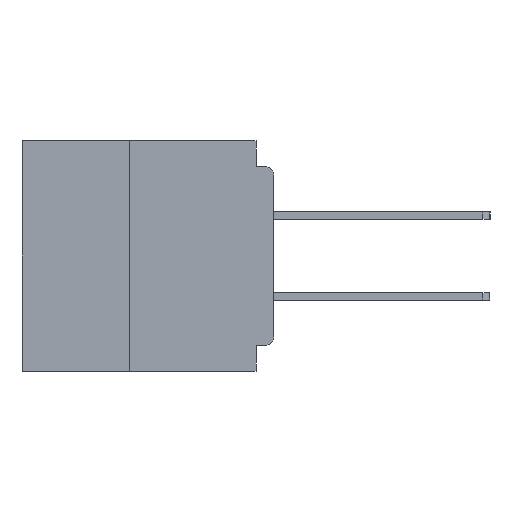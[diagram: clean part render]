
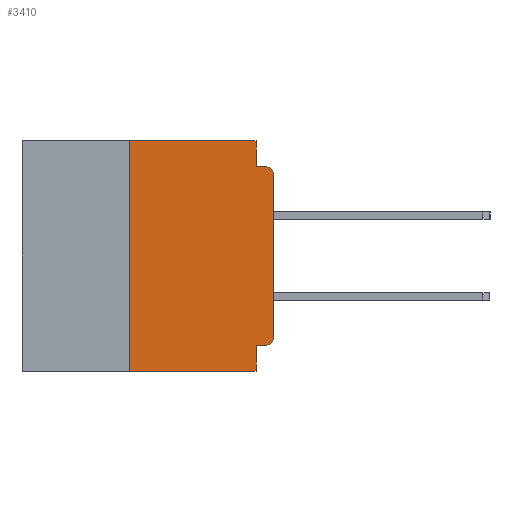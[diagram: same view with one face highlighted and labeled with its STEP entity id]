
A CAD part, left-side view. The second image highlights one B-rep face of the part: STEP entity #3410.
In plain terms, the highlighted planar face has unit normal (-1, 0, 0).
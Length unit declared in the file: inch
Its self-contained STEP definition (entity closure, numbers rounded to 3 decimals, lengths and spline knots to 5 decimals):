
#712 = EDGE_CURVE ( 'NONE', #41883, #41600, #4166, .T. ) ;
#961 = VERTEX_POINT ( 'NONE', #9339 ) ;
#2722 = VECTOR ( 'NONE', #60346, 39.37008 ) ;
#3410 = ADVANCED_FACE ( 'NONE', ( #14158 ), #40095, .F. ) ;
#4166 = CIRCLE ( 'NONE', #54427, 0.015 ) ;
#4264 = LINE ( 'NONE', #10552, #2722 ) ;
#5051 = CARTESIAN_POINT ( 'NONE',  ( 0., 0., -0.34 ) ) ;
#5794 = EDGE_CURVE ( 'NONE', #13918, #59047, #13014, .T. ) ;
#7141 = EDGE_LOOP ( 'NONE', ( #13657, #13725, #13972, #15127, #15291, #16642, #16858, #16979, #18380, #18443 ) ) ;
#9001 = VECTOR ( 'NONE', #41892, 39.37008 ) ;
#9339 = CARTESIAN_POINT ( 'NONE',  ( 0., 0.031, -0.045 ) ) ;
#10482 = VECTOR ( 'NONE', #23053, 39.37008 ) ;
#10552 = CARTESIAN_POINT ( 'NONE',  ( 0., 0., -0.045 ) ) ;
#12999 = CARTESIAN_POINT ( 'NONE',  ( 0., 0., 0. ) ) ;
#13014 = LINE ( 'NONE', #35669, #51040 ) ;
#13310 = CARTESIAN_POINT ( 'NONE',  ( 0., 0.437, 0. ) ) ;
#13657 = ORIENTED_EDGE ( 'NONE', *, *, #55321, .T. ) ;
#13725 = ORIENTED_EDGE ( 'NONE', *, *, #25751, .T. ) ;
#13918 = VERTEX_POINT ( 'NONE', #22809 ) ;
#13972 = ORIENTED_EDGE ( 'NONE', *, *, #45999, .F. ) ;
#14158 = FACE_OUTER_BOUND ( 'NONE', #7141, .T. ) ;
#14309 = CARTESIAN_POINT ( 'NONE',  ( 0., 0.25, -0.4 ) ) ;
#15127 = ORIENTED_EDGE ( 'NONE', *, *, #40998, .F. ) ;
#15291 = ORIENTED_EDGE ( 'NONE', *, *, #24713, .F. ) ;
#16642 = ORIENTED_EDGE ( 'NONE', *, *, #40316, .F. ) ;
#16858 = ORIENTED_EDGE ( 'NONE', *, *, #39664, .T. ) ;
#16963 = CARTESIAN_POINT ( 'NONE',  ( 0., 0.015, -0.355 ) ) ;
#16979 = ORIENTED_EDGE ( 'NONE', *, *, #5794, .F. ) ;
#17107 = CARTESIAN_POINT ( 'NONE',  ( 0., 0., -0.355 ) ) ;
#18256 = AXIS2_PLACEMENT_3D ( 'NONE', #50544, #20895, #55479 ) ;
#18380 = ORIENTED_EDGE ( 'NONE', *, *, #43912, .F. ) ;
#18443 = ORIENTED_EDGE ( 'NONE', *, *, #712, .T. ) ;
#19153 = VERTEX_POINT ( 'NONE', #29732 ) ;
#20151 = CARTESIAN_POINT ( 'NONE',  ( 0., 0.031, 0. ) ) ;
#20895 = DIRECTION ( 'NONE',  ( -1., 0., 0. ) ) ;
#21794 = VERTEX_POINT ( 'NONE', #53941 ) ;
#21853 = VECTOR ( 'NONE', #34099, 39.37008 ) ;
#22424 = VECTOR ( 'NONE', #33102, 39.37008 ) ;
#22809 = CARTESIAN_POINT ( 'NONE',  ( 0., 0.031, -0.355 ) ) ;
#23053 = DIRECTION ( 'NONE',  ( 0., 0., 1. ) ) ;
#23992 = LINE ( 'NONE', #13310, #22424 ) ;
#24713 = EDGE_CURVE ( 'NONE', #21794, #55453, #23992, .T. ) ;
#25751 = EDGE_CURVE ( 'NONE', #19153, #29662, #40828, .T. ) ;
#25863 = LINE ( 'NONE', #28375, #49073 ) ;
#28375 = CARTESIAN_POINT ( 'NONE',  ( 0., 0.437, -0.4 ) ) ;
#28702 = CARTESIAN_POINT ( 'NONE',  ( 0., 0.031, -0.4 ) ) ;
#29662 = VERTEX_POINT ( 'NONE', #58055 ) ;
#29732 = CARTESIAN_POINT ( 'NONE',  ( 0., 0., -0.06 ) ) ;
#33102 = DIRECTION ( 'NONE',  ( 0., -1., 0. ) ) ;
#34099 = DIRECTION ( 'NONE',  ( 0., 0., 1. ) ) ;
#35111 = VECTOR ( 'NONE', #59717, 39.37008 ) ;
#35508 = DIRECTION ( 'NONE',  ( 0., 0., -1. ) ) ;
#35669 = CARTESIAN_POINT ( 'NONE',  ( 0., 0.031, -0.4 ) ) ;
#36559 = DIRECTION ( 'NONE',  ( -1., 0., 0. ) ) ;
#36785 = CARTESIAN_POINT ( 'NONE',  ( 0., 0.015, -0.34 ) ) ;
#39664 = EDGE_CURVE ( 'NONE', #60904, #59047, #25863, .T. ) ;
#39886 = DIRECTION ( 'NONE',  ( 0., 0., -1. ) ) ;
#40095 = PLANE ( 'NONE',  #59916 ) ;
#40159 = CARTESIAN_POINT ( 'NONE',  ( 0., 0.437, 0. ) ) ;
#40316 = EDGE_CURVE ( 'NONE', #60904, #21794, #61272, .T. ) ;
#40650 = DIRECTION ( 'NONE',  ( 1., 0., 0. ) ) ;
#40658 = DIRECTION ( 'NONE',  ( 0., 0., -1. ) ) ;
#40828 = CIRCLE ( 'NONE', #18256, 0.015 ) ;
#40998 = EDGE_CURVE ( 'NONE', #55453, #961, #49763, .T. ) ;
#41600 = VERTEX_POINT ( 'NONE', #5051 ) ;
#41883 = VERTEX_POINT ( 'NONE', #16963 ) ;
#41892 = DIRECTION ( 'NONE',  ( 0., 1., 0. ) ) ;
#43912 = EDGE_CURVE ( 'NONE', #41883, #13918, #48583, .T. ) ;
#45999 = EDGE_CURVE ( 'NONE', #961, #29662, #4264, .T. ) ;
#48564 = CARTESIAN_POINT ( 'NONE',  ( 0., 0.031, 0. ) ) ;
#48583 = LINE ( 'NONE', #17107, #9001 ) ;
#49073 = VECTOR ( 'NONE', #58754, 39.37008 ) ;
#49763 = LINE ( 'NONE', #20151, #35111 ) ;
#50544 = CARTESIAN_POINT ( 'NONE',  ( 0., 0.015, -0.06 ) ) ;
#51040 = VECTOR ( 'NONE', #40658, 39.37008 ) ;
#53941 = CARTESIAN_POINT ( 'NONE',  ( 0., 0.25, 0. ) ) ;
#54427 = AXIS2_PLACEMENT_3D ( 'NONE', #36785, #36559, #35508 ) ;
#55321 = EDGE_CURVE ( 'NONE', #41600, #19153, #56222, .T. ) ;
#55453 = VERTEX_POINT ( 'NONE', #48564 ) ;
#55479 = DIRECTION ( 'NONE',  ( 0., 0., -1. ) ) ;
#56222 = LINE ( 'NONE', #12999, #10482 ) ;
#56428 = CARTESIAN_POINT ( 'NONE',  ( 0., 0.25, -0.4 ) ) ;
#58055 = CARTESIAN_POINT ( 'NONE',  ( 0., 0.015, -0.045 ) ) ;
#58754 = DIRECTION ( 'NONE',  ( 0., -1., 0. ) ) ;
#59047 = VERTEX_POINT ( 'NONE', #28702 ) ;
#59717 = DIRECTION ( 'NONE',  ( 0., 0., -1. ) ) ;
#59916 = AXIS2_PLACEMENT_3D ( 'NONE', #40159, #40650, #39886 ) ;
#60346 = DIRECTION ( 'NONE',  ( 0., -1., 0. ) ) ;
#60904 = VERTEX_POINT ( 'NONE', #56428 ) ;
#61272 = LINE ( 'NONE', #14309, #21853 ) ;
